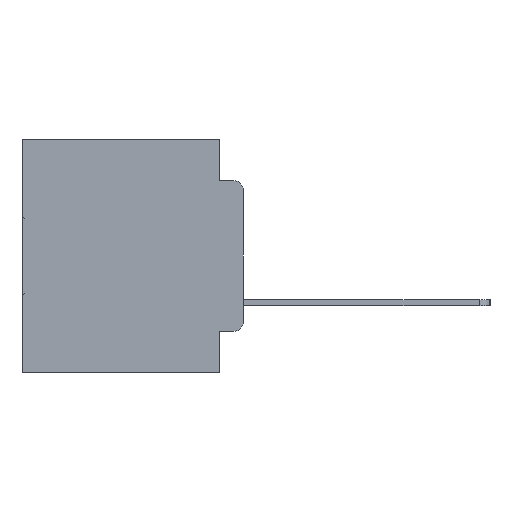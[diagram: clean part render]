
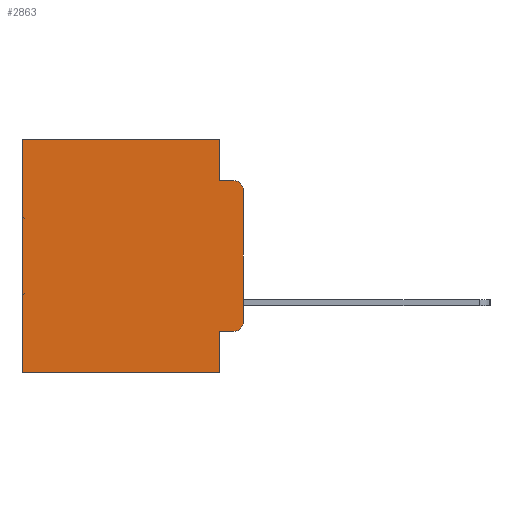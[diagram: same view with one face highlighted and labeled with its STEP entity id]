
A CAD part, left-side view. The second image highlights one B-rep face of the part: STEP entity #2863.
In plain terms, the highlighted planar face has unit normal (-1, 0, 0).
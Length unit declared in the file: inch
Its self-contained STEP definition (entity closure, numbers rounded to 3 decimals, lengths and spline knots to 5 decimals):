
#229 = AXIS2_PLACEMENT_3D ( 'NONE', #13357, #31520, #16000 ) ;
#449 = DIRECTION ( 'NONE',  ( 0., 0., -1. ) ) ;
#1261 = LINE ( 'NONE', #14449, #21576 ) ;
#2731 = ORIENTED_EDGE ( 'NONE', *, *, #11465, .T. ) ;
#2863 = ADVANCED_FACE ( 'NONE', ( #6799 ), #21101, .F. ) ;
#3325 = CARTESIAN_POINT ( 'NONE',  ( 0.298, 0., -0.5 ) ) ;
#3870 = VECTOR ( 'NONE', #22737, 39.37008 ) ;
#4008 = CARTESIAN_POINT ( 'NONE',  ( 0.298, 0.051, -0.5 ) ) ;
#4702 = VERTEX_POINT ( 'NONE', #20404 ) ;
#5304 = CARTESIAN_POINT ( 'NONE',  ( 0.298, 0., 0. ) ) ;
#5589 = LINE ( 'NONE', #3325, #26534 ) ;
#5927 = VERTEX_POINT ( 'NONE', #28366 ) ;
#6082 = ORIENTED_EDGE ( 'NONE', *, *, #26677, .T. ) ;
#6799 = FACE_OUTER_BOUND ( 'NONE', #22126, .T. ) ;
#6963 = CARTESIAN_POINT ( 'NONE',  ( 0.298, 0., 0. ) ) ;
#6997 = ORIENTED_EDGE ( 'NONE', *, *, #32561, .F. ) ;
#8019 = DIRECTION ( 'NONE',  ( 1., 0., 0. ) ) ;
#8738 = CARTESIAN_POINT ( 'NONE',  ( 0.298, 0.051, 0. ) ) ;
#9023 = LINE ( 'NONE', #8738, #14318 ) ;
#9159 = EDGE_CURVE ( 'NONE', #32973, #11026, #9023, .T. ) ;
#9919 = VERTEX_POINT ( 'NONE', #22667 ) ;
#9934 = CARTESIAN_POINT ( 'NONE',  ( 0.298, 0.051, -0.4115 ) ) ;
#10471 = VERTEX_POINT ( 'NONE', #19611 ) ;
#10555 = EDGE_CURVE ( 'NONE', #28970, #9919, #17924, .T. ) ;
#11026 = VERTEX_POINT ( 'NONE', #4008 ) ;
#11465 = EDGE_CURVE ( 'NONE', #9919, #10471, #17491, .T. ) ;
#11485 = VECTOR ( 'NONE', #32895, 39.37008 ) ;
#12213 = EDGE_CURVE ( 'NONE', #21209, #5927, #1261, .T. ) ;
#12557 = DIRECTION ( 'NONE',  ( -1., 0., 0. ) ) ;
#12604 = CARTESIAN_POINT ( 'NONE',  ( 0.298, 0.051, -0.0885 ) ) ;
#12663 = EDGE_CURVE ( 'NONE', #32973, #31952, #20714, .T. ) ;
#13264 = CIRCLE ( 'NONE', #32333, 0.02 ) ;
#13338 = AXIS2_PLACEMENT_3D ( 'NONE', #5304, #8019, #26322 ) ;
#13357 = CARTESIAN_POINT ( 'NONE',  ( 0.298, 0.02, -0.3915 ) ) ;
#14256 = CARTESIAN_POINT ( 'NONE',  ( 0.298, 0., -0.1085 ) ) ;
#14318 = VECTOR ( 'NONE', #29559, 39.37008 ) ;
#14449 = CARTESIAN_POINT ( 'NONE',  ( 0.298, 0., 0. ) ) ;
#16000 = DIRECTION ( 'NONE',  ( 0., 0., -1. ) ) ;
#16156 = EDGE_CURVE ( 'NONE', #31952, #5927, #26397, .T. ) ;
#17093 = DIRECTION ( 'NONE',  ( 0., 0., -1. ) ) ;
#17491 = LINE ( 'NONE', #21878, #31271 ) ;
#17716 = DIRECTION ( 'NONE',  ( 0., -1., 0. ) ) ;
#17924 = LINE ( 'NONE', #6963, #3870 ) ;
#18601 = CARTESIAN_POINT ( 'NONE',  ( 0.298, 0.02, -0.0885 ) ) ;
#19611 = CARTESIAN_POINT ( 'NONE',  ( 0.298, 0.473, -0.5 ) ) ;
#19650 = ORIENTED_EDGE ( 'NONE', *, *, #19677, .F. ) ;
#19677 = EDGE_CURVE ( 'NONE', #4702, #20487, #32608, .T. ) ;
#20404 = CARTESIAN_POINT ( 'NONE',  ( 0.298, 0.051, -0.0885 ) ) ;
#20487 = VERTEX_POINT ( 'NONE', #18601 ) ;
#20540 = DIRECTION ( 'NONE',  ( 0., -1., 0. ) ) ;
#20714 = LINE ( 'NONE', #9934, #27598 ) ;
#21101 = PLANE ( 'NONE',  #13338 ) ;
#21209 = VERTEX_POINT ( 'NONE', #14256 ) ;
#21576 = VECTOR ( 'NONE', #17093, 39.37008 ) ;
#21878 = CARTESIAN_POINT ( 'NONE',  ( 0.298, 0.473, 0. ) ) ;
#22126 = EDGE_LOOP ( 'NONE', ( #32594, #6082, #19650, #29763, #28205, #2731, #6997, #29450, #22651, #31056 ) ) ;
#22651 = ORIENTED_EDGE ( 'NONE', *, *, #12663, .T. ) ;
#22667 = CARTESIAN_POINT ( 'NONE',  ( 0.298, 0.473, 0. ) ) ;
#22737 = DIRECTION ( 'NONE',  ( 0., 1., 0. ) ) ;
#25816 = VECTOR ( 'NONE', #20540, 39.37008 ) ;
#26078 = CARTESIAN_POINT ( 'NONE',  ( 0.298, 0.051, -0.4115 ) ) ;
#26322 = DIRECTION ( 'NONE',  ( 0., 0., -1. ) ) ;
#26397 = CIRCLE ( 'NONE', #229, 0.02 ) ;
#26534 = VECTOR ( 'NONE', #29424, 39.37008 ) ;
#26677 = EDGE_CURVE ( 'NONE', #21209, #20487, #13264, .T. ) ;
#27598 = VECTOR ( 'NONE', #17716, 39.37008 ) ;
#27620 = CARTESIAN_POINT ( 'NONE',  ( 0.298, 0.051, 0. ) ) ;
#28193 = CARTESIAN_POINT ( 'NONE',  ( 0.298, 0.02, -0.1085 ) ) ;
#28205 = ORIENTED_EDGE ( 'NONE', *, *, #10555, .T. ) ;
#28366 = CARTESIAN_POINT ( 'NONE',  ( 0.298, 0., -0.3915 ) ) ;
#28390 = EDGE_CURVE ( 'NONE', #28970, #4702, #33047, .T. ) ;
#28970 = VERTEX_POINT ( 'NONE', #32621 ) ;
#29424 = DIRECTION ( 'NONE',  ( 0., 1., 0. ) ) ;
#29450 = ORIENTED_EDGE ( 'NONE', *, *, #9159, .F. ) ;
#29559 = DIRECTION ( 'NONE',  ( 0., 0., -1. ) ) ;
#29763 = ORIENTED_EDGE ( 'NONE', *, *, #28390, .F. ) ;
#30716 = DIRECTION ( 'NONE',  ( 0., 0., -1. ) ) ;
#31056 = ORIENTED_EDGE ( 'NONE', *, *, #16156, .T. ) ;
#31271 = VECTOR ( 'NONE', #449, 39.37008 ) ;
#31520 = DIRECTION ( 'NONE',  ( -1., 0., 0. ) ) ;
#31952 = VERTEX_POINT ( 'NONE', #33934 ) ;
#32333 = AXIS2_PLACEMENT_3D ( 'NONE', #28193, #12557, #30716 ) ;
#32561 = EDGE_CURVE ( 'NONE', #11026, #10471, #5589, .T. ) ;
#32594 = ORIENTED_EDGE ( 'NONE', *, *, #12213, .F. ) ;
#32608 = LINE ( 'NONE', #12604, #25816 ) ;
#32621 = CARTESIAN_POINT ( 'NONE',  ( 0.298, 0.051, 0. ) ) ;
#32895 = DIRECTION ( 'NONE',  ( 0., 0., -1. ) ) ;
#32973 = VERTEX_POINT ( 'NONE', #26078 ) ;
#33047 = LINE ( 'NONE', #27620, #11485 ) ;
#33934 = CARTESIAN_POINT ( 'NONE',  ( 0.298, 0.02, -0.4115 ) ) ;
